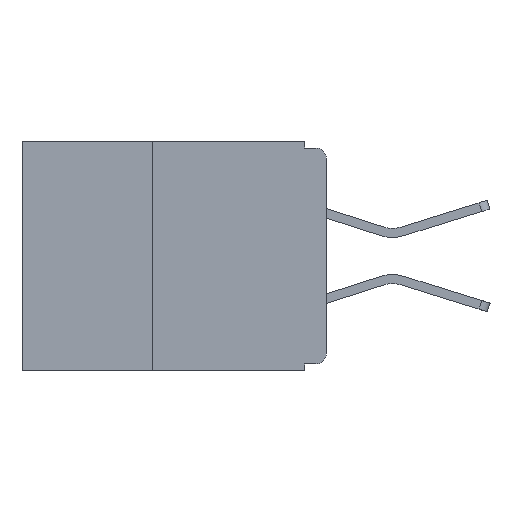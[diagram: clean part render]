
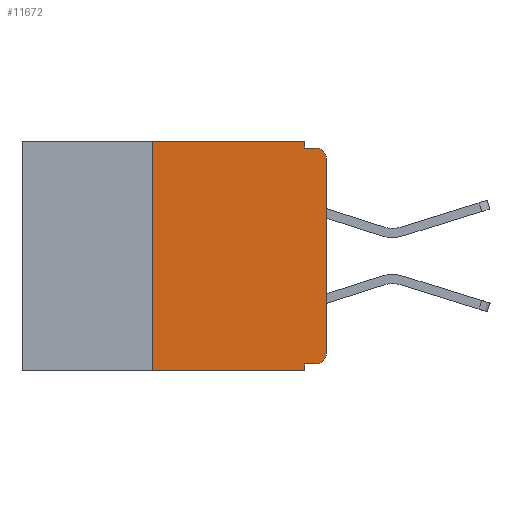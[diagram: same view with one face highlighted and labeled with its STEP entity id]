
A CAD part, left-side view. The second image highlights one B-rep face of the part: STEP entity #11672.
In plain terms, the highlighted planar face has unit normal (-1, 0, 0).
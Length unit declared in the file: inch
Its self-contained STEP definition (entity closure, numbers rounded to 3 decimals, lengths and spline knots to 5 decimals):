
#148 = ORIENTED_EDGE ( 'NONE', *, *, #3072, .T. ) ;
#317 = PLANE ( 'NONE',  #9777 ) ;
#341 = DIRECTION ( 'NONE',  ( 0., 0., -1. ) ) ;
#401 = CARTESIAN_POINT ( 'NONE',  ( 0., 0.015, -0.025 ) ) ;
#739 = CARTESIAN_POINT ( 'NONE',  ( 0., 0.031, 0. ) ) ;
#931 = VECTOR ( 'NONE', #12119, 39.37008 ) ;
#1239 = DIRECTION ( 'NONE',  ( 0., 0., -1. ) ) ;
#1647 = VERTEX_POINT ( 'NONE', #13954 ) ;
#1760 = EDGE_CURVE ( 'NONE', #8850, #6332, #10061, .T. ) ;
#1829 = VECTOR ( 'NONE', #1239, 39.37008 ) ;
#1839 = AXIS2_PLACEMENT_3D ( 'NONE', #401, #8410, #341 ) ;
#2110 = DIRECTION ( 'NONE',  ( 0., -1., 0. ) ) ;
#2196 = LINE ( 'NONE', #3424, #1829 ) ;
#2497 = CARTESIAN_POINT ( 'NONE',  ( 0., 0.25, -0.33 ) ) ;
#2625 = CARTESIAN_POINT ( 'NONE',  ( 0., 0.437, 0. ) ) ;
#2784 = VERTEX_POINT ( 'NONE', #7783 ) ;
#3072 = EDGE_CURVE ( 'NONE', #8949, #10259, #11724, .T. ) ;
#3206 = VERTEX_POINT ( 'NONE', #5238 ) ;
#3424 = CARTESIAN_POINT ( 'NONE',  ( 0., 0.031, -0.33 ) ) ;
#3645 = DIRECTION ( 'NONE',  ( 0., 0., 1. ) ) ;
#3844 = CARTESIAN_POINT ( 'NONE',  ( 0., 0., 0. ) ) ;
#4102 = ORIENTED_EDGE ( 'NONE', *, *, #11504, .F. ) ;
#4176 = VECTOR ( 'NONE', #11138, 39.37008 ) ;
#4211 = EDGE_CURVE ( 'NONE', #14175, #8949, #12231, .T. ) ;
#4301 = CARTESIAN_POINT ( 'NONE',  ( 0., 0., -0.025 ) ) ;
#4431 = VECTOR ( 'NONE', #2110, 39.37008 ) ;
#4724 = ORIENTED_EDGE ( 'NONE', *, *, #12474, .F. ) ;
#4919 = VECTOR ( 'NONE', #3645, 39.37008 ) ;
#4959 = CIRCLE ( 'NONE', #1839, 0.015 ) ;
#5238 = CARTESIAN_POINT ( 'NONE',  ( 0., 0.015, -0.01 ) ) ;
#5360 = ORIENTED_EDGE ( 'NONE', *, *, #4211, .T. ) ;
#5696 = VECTOR ( 'NONE', #11033, 39.37008 ) ;
#5728 = FACE_OUTER_BOUND ( 'NONE', #11529, .T. ) ;
#5966 = ORIENTED_EDGE ( 'NONE', *, *, #6989, .F. ) ;
#6035 = DIRECTION ( 'NONE',  ( 1., 0., 0. ) ) ;
#6206 = ORIENTED_EDGE ( 'NONE', *, *, #9446, .F. ) ;
#6332 = VERTEX_POINT ( 'NONE', #7637 ) ;
#6932 = CARTESIAN_POINT ( 'NONE',  ( 0., 0.031, -0.01 ) ) ;
#6989 = EDGE_CURVE ( 'NONE', #14175, #1647, #12148, .T. ) ;
#7637 = CARTESIAN_POINT ( 'NONE',  ( 0., 0.031, -0.33 ) ) ;
#7719 = LINE ( 'NONE', #739, #931 ) ;
#7783 = CARTESIAN_POINT ( 'NONE',  ( 0., 0.031, 0. ) ) ;
#8025 = ORIENTED_EDGE ( 'NONE', *, *, #8258, .F. ) ;
#8250 = ORIENTED_EDGE ( 'NONE', *, *, #1760, .T. ) ;
#8258 = EDGE_CURVE ( 'NONE', #9836, #3206, #12802, .T. ) ;
#8410 = DIRECTION ( 'NONE',  ( -1., 0., 0. ) ) ;
#8821 = ORIENTED_EDGE ( 'NONE', *, *, #10236, .F. ) ;
#8850 = VERTEX_POINT ( 'NONE', #11834 ) ;
#8931 = CARTESIAN_POINT ( 'NONE',  ( 0., 0.25, 0. ) ) ;
#8949 = VERTEX_POINT ( 'NONE', #14233 ) ;
#9088 = VECTOR ( 'NONE', #14737, 39.37008 ) ;
#9446 = EDGE_CURVE ( 'NONE', #8850, #10280, #14003, .T. ) ;
#9777 = AXIS2_PLACEMENT_3D ( 'NONE', #2625, #6035, #14008 ) ;
#9836 = VERTEX_POINT ( 'NONE', #6932 ) ;
#10025 = CARTESIAN_POINT ( 'NONE',  ( 0., 0.437, 0. ) ) ;
#10050 = CARTESIAN_POINT ( 'NONE',  ( 0., 0., -0.01 ) ) ;
#10061 = LINE ( 'NONE', #10692, #13049 ) ;
#10236 = EDGE_CURVE ( 'NONE', #10280, #2784, #13263, .T. ) ;
#10259 = VERTEX_POINT ( 'NONE', #4301 ) ;
#10280 = VERTEX_POINT ( 'NONE', #8931 ) ;
#10652 = DIRECTION ( 'NONE',  ( 0., 0., -1. ) ) ;
#10661 = DIRECTION ( 'NONE',  ( -1., 0., 0. ) ) ;
#10663 = DIRECTION ( 'NONE',  ( 0., -1., 0. ) ) ;
#10667 = CARTESIAN_POINT ( 'NONE',  ( 0., 0.015, -0.305 ) ) ;
#10692 = CARTESIAN_POINT ( 'NONE',  ( 0., 0.437, -0.33 ) ) ;
#10993 = ORIENTED_EDGE ( 'NONE', *, *, #14121, .T. ) ;
#11033 = DIRECTION ( 'NONE',  ( 0., 1., 0. ) ) ;
#11138 = DIRECTION ( 'NONE',  ( 0., -1., 0. ) ) ;
#11504 = EDGE_CURVE ( 'NONE', #1647, #6332, #2196, .T. ) ;
#11529 = EDGE_LOOP ( 'NONE', ( #148, #10993, #8025, #4724, #8821, #6206, #8250, #4102, #5966, #5360 ) ) ;
#11672 = ADVANCED_FACE ( 'NONE', ( #5728 ), #317, .F. ) ;
#11724 = LINE ( 'NONE', #3844, #9088 ) ;
#11834 = CARTESIAN_POINT ( 'NONE',  ( 0., 0.25, -0.33 ) ) ;
#12119 = DIRECTION ( 'NONE',  ( 0., 0., -1. ) ) ;
#12148 = LINE ( 'NONE', #12205, #5696 ) ;
#12205 = CARTESIAN_POINT ( 'NONE',  ( 0., 0., -0.32 ) ) ;
#12231 = CIRCLE ( 'NONE', #14540, 0.015 ) ;
#12474 = EDGE_CURVE ( 'NONE', #2784, #9836, #7719, .T. ) ;
#12802 = LINE ( 'NONE', #10050, #4431 ) ;
#13049 = VECTOR ( 'NONE', #10663, 39.37008 ) ;
#13263 = LINE ( 'NONE', #10025, #4176 ) ;
#13740 = CARTESIAN_POINT ( 'NONE',  ( 0., 0.015, -0.32 ) ) ;
#13954 = CARTESIAN_POINT ( 'NONE',  ( 0., 0.031, -0.32 ) ) ;
#14003 = LINE ( 'NONE', #2497, #4919 ) ;
#14008 = DIRECTION ( 'NONE',  ( 0., 0., -1. ) ) ;
#14121 = EDGE_CURVE ( 'NONE', #10259, #3206, #4959, .T. ) ;
#14175 = VERTEX_POINT ( 'NONE', #13740 ) ;
#14233 = CARTESIAN_POINT ( 'NONE',  ( 0., 0., -0.305 ) ) ;
#14540 = AXIS2_PLACEMENT_3D ( 'NONE', #10667, #10661, #10652 ) ;
#14737 = DIRECTION ( 'NONE',  ( 0., 0., 1. ) ) ;
